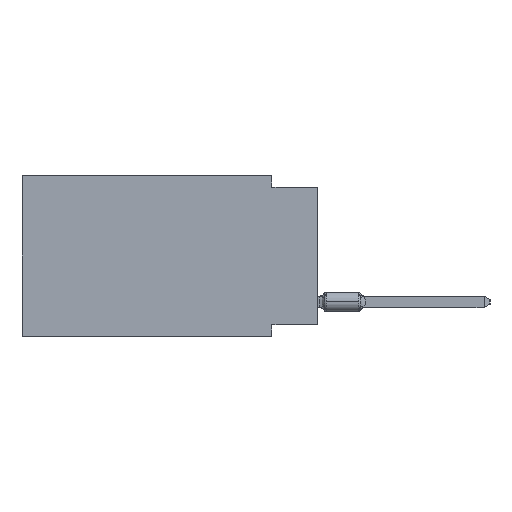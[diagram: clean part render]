
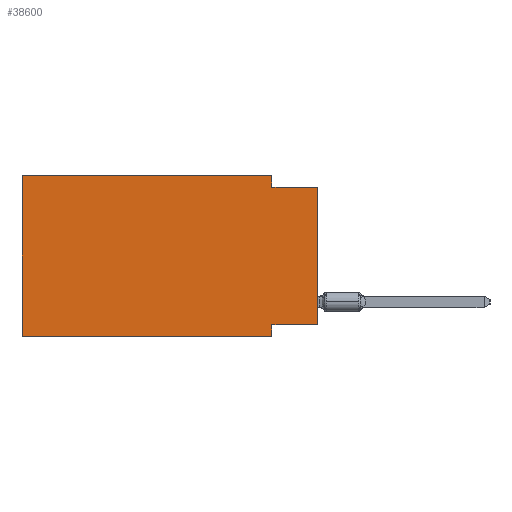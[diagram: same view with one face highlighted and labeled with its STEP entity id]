
A CAD part, left-side view. The second image highlights one B-rep face of the part: STEP entity #38600.
In plain terms, the highlighted planar face has unit normal (-1, 0, 0).
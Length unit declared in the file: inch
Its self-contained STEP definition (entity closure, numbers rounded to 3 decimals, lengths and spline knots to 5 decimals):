
#778 = DIRECTION ( 'NONE',  ( 0., -1., 0. ) ) ;
#802 = VERTEX_POINT ( 'NONE', #11032 ) ;
#886 = ORIENTED_EDGE ( 'NONE', *, *, #27283, .F. ) ;
#1048 = LINE ( 'NONE', #31988, #22283 ) ;
#1259 = CARTESIAN_POINT ( 'NONE',  ( 0., 0.1, -0.025 ) ) ;
#1899 = DIRECTION ( 'NONE',  ( 0., -1., 0. ) ) ;
#1943 = PLANE ( 'NONE',  #29266 ) ;
#2286 = DIRECTION ( 'NONE',  ( 0., 0., 1. ) ) ;
#3074 = CARTESIAN_POINT ( 'NONE',  ( 0., 0.645, 0. ) ) ;
#3299 = ORIENTED_EDGE ( 'NONE', *, *, #30215, .F. ) ;
#4063 = DIRECTION ( 'NONE',  ( 0., 0., 1. ) ) ;
#5296 = LINE ( 'NONE', #29825, #13056 ) ;
#5462 = ORIENTED_EDGE ( 'NONE', *, *, #7952, .F. ) ;
#5691 = EDGE_CURVE ( 'NONE', #33075, #15977, #1048, .T. ) ;
#6793 = LINE ( 'NONE', #16431, #19504 ) ;
#7952 = EDGE_CURVE ( 'NONE', #39753, #14774, #37036, .T. ) ;
#8134 = CARTESIAN_POINT ( 'NONE',  ( 0., 0., -0.025 ) ) ;
#9007 = DIRECTION ( 'NONE',  ( 0., 0., -1. ) ) ;
#10303 = CARTESIAN_POINT ( 'NONE',  ( 0., 0.645, 0. ) ) ;
#11032 = CARTESIAN_POINT ( 'NONE',  ( 0., 0., -0.025 ) ) ;
#11822 = VECTOR ( 'NONE', #32940, 39.37008 ) ;
#12112 = EDGE_CURVE ( 'NONE', #37923, #22541, #6793, .T. ) ;
#12226 = LINE ( 'NONE', #24273, #28327 ) ;
#13056 = VECTOR ( 'NONE', #2286, 39.37008 ) ;
#13092 = ORIENTED_EDGE ( 'NONE', *, *, #5691, .F. ) ;
#14546 = ORIENTED_EDGE ( 'NONE', *, *, #12112, .T. ) ;
#14774 = VERTEX_POINT ( 'NONE', #34058 ) ;
#15952 = LINE ( 'NONE', #10303, #18005 ) ;
#15977 = VERTEX_POINT ( 'NONE', #33733 ) ;
#16431 = CARTESIAN_POINT ( 'NONE',  ( 0., 0.645, -0.35 ) ) ;
#18005 = VECTOR ( 'NONE', #4063, 39.37008 ) ;
#19129 = DIRECTION ( 'NONE',  ( 0., 1., 0. ) ) ;
#19492 = CARTESIAN_POINT ( 'NONE',  ( 0., 0.645, 0. ) ) ;
#19504 = VECTOR ( 'NONE', #778, 39.37008 ) ;
#20082 = EDGE_LOOP ( 'NONE', ( #31252, #886, #27944, #5462, #23689, #14546, #3299, #13092 ) ) ;
#20837 = CARTESIAN_POINT ( 'NONE',  ( 0., 0.645, 0. ) ) ;
#21147 = EDGE_CURVE ( 'NONE', #37923, #39753, #15952, .T. ) ;
#21642 = VERTEX_POINT ( 'NONE', #1259 ) ;
#22283 = VECTOR ( 'NONE', #19129, 39.37008 ) ;
#22324 = EDGE_CURVE ( 'NONE', #14774, #21642, #12226, .T. ) ;
#22541 = VERTEX_POINT ( 'NONE', #23415 ) ;
#23415 = CARTESIAN_POINT ( 'NONE',  ( 0., 0.1, -0.35 ) ) ;
#23682 = LINE ( 'NONE', #35753, #11822 ) ;
#23689 = ORIENTED_EDGE ( 'NONE', *, *, #21147, .F. ) ;
#23806 = LINE ( 'NONE', #8134, #27706 ) ;
#24273 = CARTESIAN_POINT ( 'NONE',  ( 0., 0.1, 0. ) ) ;
#26342 = CARTESIAN_POINT ( 'NONE',  ( 0., 0., -0.325 ) ) ;
#27204 = DIRECTION ( 'NONE',  ( 0., -1., 0. ) ) ;
#27283 = EDGE_CURVE ( 'NONE', #21642, #802, #23806, .T. ) ;
#27706 = VECTOR ( 'NONE', #1899, 39.37008 ) ;
#27944 = ORIENTED_EDGE ( 'NONE', *, *, #22324, .F. ) ;
#28327 = VECTOR ( 'NONE', #9007, 39.37008 ) ;
#29266 = AXIS2_PLACEMENT_3D ( 'NONE', #20837, #38530, #38734 ) ;
#29825 = CARTESIAN_POINT ( 'NONE',  ( 0., 0., 0. ) ) ;
#29958 = EDGE_CURVE ( 'NONE', #33075, #802, #5296, .T. ) ;
#30215 = EDGE_CURVE ( 'NONE', #15977, #22541, #23682, .T. ) ;
#30768 = VECTOR ( 'NONE', #27204, 39.37008 ) ;
#31252 = ORIENTED_EDGE ( 'NONE', *, *, #29958, .T. ) ;
#31988 = CARTESIAN_POINT ( 'NONE',  ( 0., 0., -0.325 ) ) ;
#32940 = DIRECTION ( 'NONE',  ( 0., 0., -1. ) ) ;
#33075 = VERTEX_POINT ( 'NONE', #26342 ) ;
#33733 = CARTESIAN_POINT ( 'NONE',  ( 0., 0.1, -0.325 ) ) ;
#34058 = CARTESIAN_POINT ( 'NONE',  ( 0., 0.1, 0. ) ) ;
#35514 = FACE_OUTER_BOUND ( 'NONE', #20082, .T. ) ;
#35753 = CARTESIAN_POINT ( 'NONE',  ( 0., 0.1, -0.35 ) ) ;
#37036 = LINE ( 'NONE', #3074, #30768 ) ;
#37923 = VERTEX_POINT ( 'NONE', #38471 ) ;
#38471 = CARTESIAN_POINT ( 'NONE',  ( 0., 0.645, -0.35 ) ) ;
#38530 = DIRECTION ( 'NONE',  ( 1., 0., 0. ) ) ;
#38600 = ADVANCED_FACE ( 'NONE', ( #35514 ), #1943, .F. ) ;
#38734 = DIRECTION ( 'NONE',  ( 0., 0., -1. ) ) ;
#39753 = VERTEX_POINT ( 'NONE', #19492 ) ;
